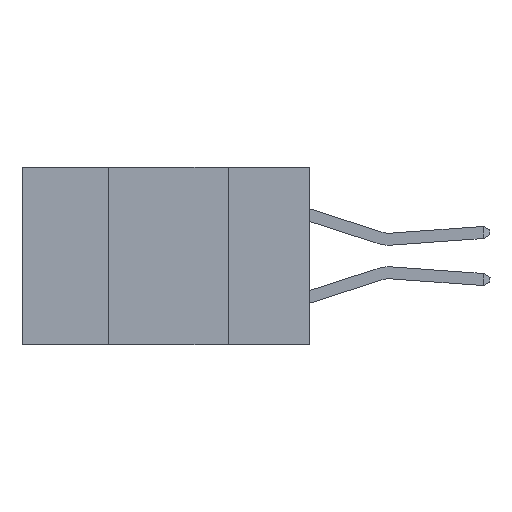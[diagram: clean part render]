
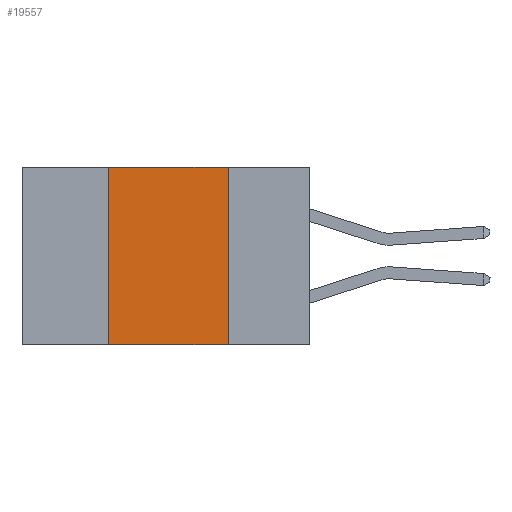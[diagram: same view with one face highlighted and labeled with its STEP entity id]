
A CAD part, left-side view. The second image highlights one B-rep face of the part: STEP entity #19557.
In plain terms, the highlighted planar face has unit normal (-1, 0, 0).
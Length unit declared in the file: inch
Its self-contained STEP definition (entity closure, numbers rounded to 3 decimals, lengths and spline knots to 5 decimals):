
#992 = CARTESIAN_POINT ( 'NONE',  ( 0., 0.6, 0. ) ) ;
#1478 = LINE ( 'NONE', #9434, #17907 ) ;
#1761 = DIRECTION ( 'NONE',  ( 0., 0., 1. ) ) ;
#1970 = VECTOR ( 'NONE', #1761, 39.37008 ) ;
#2516 = CARTESIAN_POINT ( 'NONE',  ( 0., 0.17, -0.37 ) ) ;
#2680 = CARTESIAN_POINT ( 'NONE',  ( 0., 0.17, 0. ) ) ;
#3619 = ORIENTED_EDGE ( 'NONE', *, *, #19545, .F. ) ;
#3721 = ORIENTED_EDGE ( 'NONE', *, *, #7661, .F. ) ;
#3761 = ORIENTED_EDGE ( 'NONE', *, *, #8481, .F. ) ;
#3782 = ORIENTED_EDGE ( 'NONE', *, *, #15455, .T. ) ;
#3982 = VERTEX_POINT ( 'NONE', #2516 ) ;
#4352 = DIRECTION ( 'NONE',  ( 0., 0., -1. ) ) ;
#5529 = VECTOR ( 'NONE', #20484, 39.37008 ) ;
#6499 = VERTEX_POINT ( 'NONE', #8913 ) ;
#7609 = PLANE ( 'NONE',  #9234 ) ;
#7661 = EDGE_CURVE ( 'NONE', #11696, #9818, #1478, .T. ) ;
#7670 = FACE_OUTER_BOUND ( 'NONE', #12221, .T. ) ;
#8481 = EDGE_CURVE ( 'NONE', #6499, #11696, #10541, .T. ) ;
#8913 = CARTESIAN_POINT ( 'NONE',  ( 0., 0.42, -0.37 ) ) ;
#9234 = AXIS2_PLACEMENT_3D ( 'NONE', #992, #20024, #10748 ) ;
#9434 = CARTESIAN_POINT ( 'NONE',  ( 0., 0.6, 0. ) ) ;
#9818 = VERTEX_POINT ( 'NONE', #10050 ) ;
#10050 = CARTESIAN_POINT ( 'NONE',  ( 0., 0.17, 0. ) ) ;
#10265 = CARTESIAN_POINT ( 'NONE',  ( 0., 0.42, 0. ) ) ;
#10541 = LINE ( 'NONE', #12953, #1970 ) ;
#10748 = DIRECTION ( 'NONE',  ( 0., 0., -1. ) ) ;
#11336 = CARTESIAN_POINT ( 'NONE',  ( 0., 0.6, -0.37 ) ) ;
#11696 = VERTEX_POINT ( 'NONE', #10265 ) ;
#12221 = EDGE_LOOP ( 'NONE', ( #3619, #3721, #3761, #3782 ) ) ;
#12953 = CARTESIAN_POINT ( 'NONE',  ( 0., 0.42, 0. ) ) ;
#13852 = LINE ( 'NONE', #11336, #5529 ) ;
#15455 = EDGE_CURVE ( 'NONE', #6499, #3982, #13852, .T. ) ;
#15761 = DIRECTION ( 'NONE',  ( 0., -1., 0. ) ) ;
#17907 = VECTOR ( 'NONE', #15761, 39.37008 ) ;
#19464 = LINE ( 'NONE', #2680, #20051 ) ;
#19545 = EDGE_CURVE ( 'NONE', #9818, #3982, #19464, .T. ) ;
#19557 = ADVANCED_FACE ( 'NONE', ( #7670 ), #7609, .F. ) ;
#20024 = DIRECTION ( 'NONE',  ( 1., 0., 0. ) ) ;
#20051 = VECTOR ( 'NONE', #4352, 39.37008 ) ;
#20484 = DIRECTION ( 'NONE',  ( 0., -1., 0. ) ) ;
